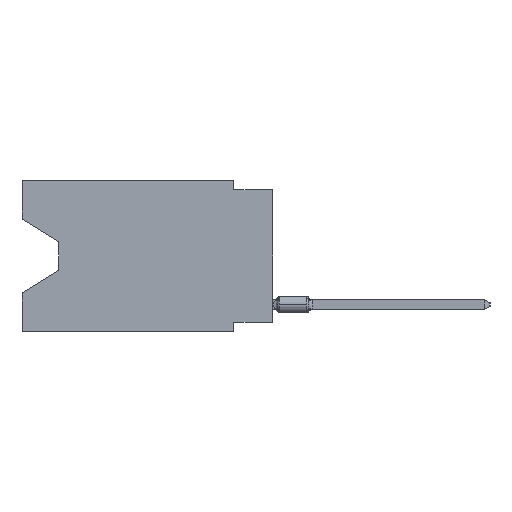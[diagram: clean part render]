
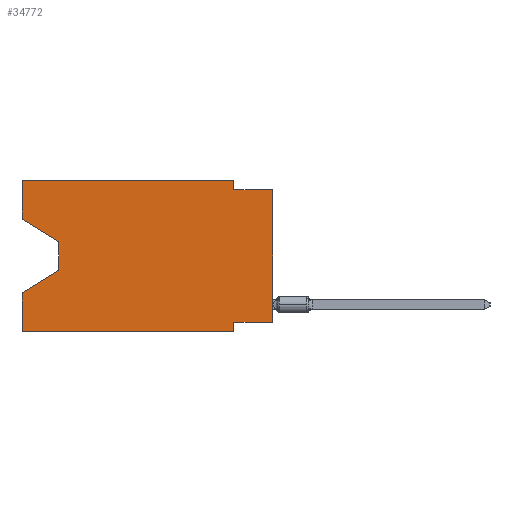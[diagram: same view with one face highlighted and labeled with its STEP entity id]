
A CAD part, left-side view. The second image highlights one B-rep face of the part: STEP entity #34772.
In plain terms, the highlighted planar face has unit normal (-1, 0, 0).
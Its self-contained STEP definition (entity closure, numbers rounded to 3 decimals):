
#508 = DIRECTION ( 'NONE',  ( 0., 1., 0. ) ) ;
#1859 = DIRECTION ( 'NONE',  ( 0., 0., 1. ) ) ;
#1874 = DIRECTION ( 'NONE',  ( 1., 0., 0. ) ) ;
#2625 = FACE_OUTER_BOUND ( 'NONE', #36561, .T. ) ;
#2905 = DIRECTION ( 'NONE',  ( 0., -0.855, -0.519 ) ) ;
#3054 = LINE ( 'NONE', #14375, #37693 ) ;
#4287 = LINE ( 'NONE', #46567, #43923 ) ;
#4533 = ORIENTED_EDGE ( 'NONE', *, *, #33437, .T. ) ;
#4914 = LINE ( 'NONE', #42429, #31337 ) ;
#5221 = DIRECTION ( 'NONE',  ( 0., 0., 1. ) ) ;
#5446 = VERTEX_POINT ( 'NONE', #36406 ) ;
#5460 = CARTESIAN_POINT ( 'NONE',  ( 0., 16.383, 0. ) ) ;
#6111 = DIRECTION ( 'NONE',  ( 0., 0., -1. ) ) ;
#6126 = DIRECTION ( 'NONE',  ( 0., 0., 1. ) ) ;
#6303 = DIRECTION ( 'NONE',  ( 0., 0., -1. ) ) ;
#6703 = VERTEX_POINT ( 'NONE', #17134 ) ;
#7468 = ORIENTED_EDGE ( 'NONE', *, *, #48800, .F. ) ;
#7524 = EDGE_CURVE ( 'NONE', #31245, #29591, #46232, .T. ) ;
#8939 = EDGE_CURVE ( 'NONE', #5446, #16403, #48480, .T. ) ;
#10635 = ORIENTED_EDGE ( 'NONE', *, *, #21434, .F. ) ;
#11099 = CARTESIAN_POINT ( 'NONE',  ( 0., 2.54, -9.906 ) ) ;
#11107 = VERTEX_POINT ( 'NONE', #22723 ) ;
#11338 = DIRECTION ( 'NONE',  ( 0., 0.855, -0.519 ) ) ;
#11460 = ORIENTED_EDGE ( 'NONE', *, *, #8939, .T. ) ;
#12190 = DIRECTION ( 'NONE',  ( 0., -1., 0. ) ) ;
#12432 = LINE ( 'NONE', #31334, #34030 ) ;
#12493 = CARTESIAN_POINT ( 'NONE',  ( 0., 0., 0. ) ) ;
#13161 = LINE ( 'NONE', #28528, #36980 ) ;
#14101 = EDGE_CURVE ( 'NONE', #39199, #21972, #29559, .T. ) ;
#14180 = PLANE ( 'NONE',  #40655 ) ;
#14375 = CARTESIAN_POINT ( 'NONE',  ( 0., 13.97, -5.893 ) ) ;
#14468 = CARTESIAN_POINT ( 'NONE',  ( 0., 2.54, -9.271 ) ) ;
#14853 = LINE ( 'NONE', #46304, #49601 ) ;
#15802 = VECTOR ( 'NONE', #23089, 1000. ) ;
#16029 = CARTESIAN_POINT ( 'NONE',  ( 0., 0., -0.635 ) ) ;
#16176 = ORIENTED_EDGE ( 'NONE', *, *, #24029, .F. ) ;
#16403 = VERTEX_POINT ( 'NONE', #30636 ) ;
#16530 = ORIENTED_EDGE ( 'NONE', *, *, #7524, .F. ) ;
#16570 = LINE ( 'NONE', #5460, #37240 ) ;
#17134 = CARTESIAN_POINT ( 'NONE',  ( 0., 13.97, -5.893 ) ) ;
#17229 = DIRECTION ( 'NONE',  ( 0., 0., -1. ) ) ;
#17699 = VECTOR ( 'NONE', #6111, 1000. ) ;
#18900 = VECTOR ( 'NONE', #6126, 1000. ) ;
#20311 = ORIENTED_EDGE ( 'NONE', *, *, #44198, .F. ) ;
#20674 = VERTEX_POINT ( 'NONE', #11099 ) ;
#20740 = ORIENTED_EDGE ( 'NONE', *, *, #39352, .T. ) ;
#21434 = EDGE_CURVE ( 'NONE', #21972, #31245, #4914, .T. ) ;
#21972 = VERTEX_POINT ( 'NONE', #35810 ) ;
#22401 = ORIENTED_EDGE ( 'NONE', *, *, #27015, .T. ) ;
#22723 = CARTESIAN_POINT ( 'NONE',  ( 0., 0., -9.271 ) ) ;
#23089 = DIRECTION ( 'NONE',  ( 0., -1., 0. ) ) ;
#24029 = EDGE_CURVE ( 'NONE', #27219, #32434, #16570, .T. ) ;
#24286 = VECTOR ( 'NONE', #2905, 1000. ) ;
#26555 = CARTESIAN_POINT ( 'NONE',  ( 0., 16.383, 0. ) ) ;
#27015 = EDGE_CURVE ( 'NONE', #11107, #29591, #47013, .T. ) ;
#27219 = VERTEX_POINT ( 'NONE', #46641 ) ;
#27755 = CARTESIAN_POINT ( 'NONE',  ( 0., 2.54, -0.635 ) ) ;
#27972 = VECTOR ( 'NONE', #37127, 1000. ) ;
#28528 = CARTESIAN_POINT ( 'NONE',  ( 0., 16.383, 0. ) ) ;
#29061 = CARTESIAN_POINT ( 'NONE',  ( 0., 16.383, 0. ) ) ;
#29559 = LINE ( 'NONE', #29061, #27972 ) ;
#29591 = VERTEX_POINT ( 'NONE', #38910 ) ;
#30636 = CARTESIAN_POINT ( 'NONE',  ( 0., 13.97, -4.013 ) ) ;
#31245 = VERTEX_POINT ( 'NONE', #27755 ) ;
#31334 = CARTESIAN_POINT ( 'NONE',  ( 0., 16.383, -9.906 ) ) ;
#31337 = VECTOR ( 'NONE', #31346, 1000. ) ;
#31346 = DIRECTION ( 'NONE',  ( 0., 0., -1. ) ) ;
#32344 = ORIENTED_EDGE ( 'NONE', *, *, #39424, .F. ) ;
#32434 = VERTEX_POINT ( 'NONE', #41081 ) ;
#33437 = EDGE_CURVE ( 'NONE', #27219, #20674, #12432, .T. ) ;
#33583 = CARTESIAN_POINT ( 'NONE',  ( 0., 16.383, 0. ) ) ;
#33866 = CARTESIAN_POINT ( 'NONE',  ( 0., 16.383, -2.546 ) ) ;
#34030 = VECTOR ( 'NONE', #12190, 1000. ) ;
#34772 = ADVANCED_FACE ( 'NONE', ( #2625 ), #14180, .F. ) ;
#35810 = CARTESIAN_POINT ( 'NONE',  ( 0., 2.54, 0. ) ) ;
#36406 = CARTESIAN_POINT ( 'NONE',  ( 0., 16.383, -2.546 ) ) ;
#36539 = ORIENTED_EDGE ( 'NONE', *, *, #45706, .T. ) ;
#36561 = EDGE_LOOP ( 'NONE', ( #11460, #20740, #36539, #16176, #4533, #20311, #7468, #22401, #16530, #10635, #43225, #32344 ) ) ;
#36980 = VECTOR ( 'NONE', #1859, 1000. ) ;
#37127 = DIRECTION ( 'NONE',  ( 0., -1., 0. ) ) ;
#37240 = VECTOR ( 'NONE', #5221, 1000. ) ;
#37693 = VECTOR ( 'NONE', #11338, 1000. ) ;
#37973 = VERTEX_POINT ( 'NONE', #14468 ) ;
#38910 = CARTESIAN_POINT ( 'NONE',  ( 0., 0., -0.635 ) ) ;
#39199 = VERTEX_POINT ( 'NONE', #26555 ) ;
#39352 = EDGE_CURVE ( 'NONE', #16403, #6703, #40366, .T. ) ;
#39424 = EDGE_CURVE ( 'NONE', #5446, #39199, #13161, .T. ) ;
#40366 = LINE ( 'NONE', #48431, #17699 ) ;
#40655 = AXIS2_PLACEMENT_3D ( 'NONE', #33583, #1874, #17229 ) ;
#41081 = CARTESIAN_POINT ( 'NONE',  ( 0., 16.383, -7.36 ) ) ;
#42429 = CARTESIAN_POINT ( 'NONE',  ( 0., 2.54, 0. ) ) ;
#43225 = ORIENTED_EDGE ( 'NONE', *, *, #14101, .F. ) ;
#43923 = VECTOR ( 'NONE', #508, 1000. ) ;
#44198 = EDGE_CURVE ( 'NONE', #37973, #20674, #14853, .T. ) ;
#45706 = EDGE_CURVE ( 'NONE', #6703, #32434, #3054, .T. ) ;
#46232 = LINE ( 'NONE', #16029, #15802 ) ;
#46304 = CARTESIAN_POINT ( 'NONE',  ( 0., 2.54, -9.906 ) ) ;
#46567 = CARTESIAN_POINT ( 'NONE',  ( 0., 0., -9.271 ) ) ;
#46641 = CARTESIAN_POINT ( 'NONE',  ( 0., 16.383, -9.906 ) ) ;
#47013 = LINE ( 'NONE', #12493, #18900 ) ;
#48431 = CARTESIAN_POINT ( 'NONE',  ( 0., 13.97, -4.013 ) ) ;
#48480 = LINE ( 'NONE', #33866, #24286 ) ;
#48800 = EDGE_CURVE ( 'NONE', #11107, #37973, #4287, .T. ) ;
#49601 = VECTOR ( 'NONE', #6303, 1000. ) ;
